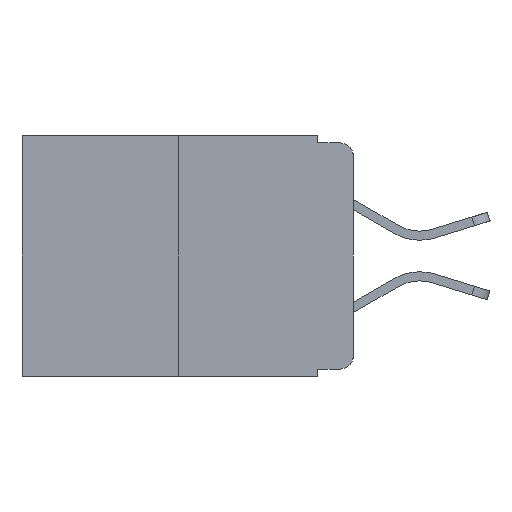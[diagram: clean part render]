
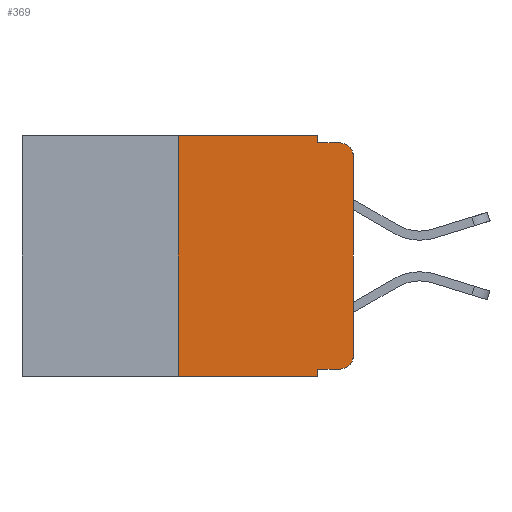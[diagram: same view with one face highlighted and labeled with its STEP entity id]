
A CAD part, left-side view. The second image highlights one B-rep face of the part: STEP entity #369.
In plain terms, the highlighted planar face has unit normal (-1, 0, 0).
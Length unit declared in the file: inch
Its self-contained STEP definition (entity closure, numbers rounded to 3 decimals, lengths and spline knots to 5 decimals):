
#134 = VERTEX_POINT ( 'NONE', #165 ) ;
#165 = CARTESIAN_POINT ( 'NONE',  ( 0., 0.051, 0. ) ) ;
#369 = ADVANCED_FACE ( 'NONE', ( #11028 ), #12728, .F. ) ;
#569 = LINE ( 'NONE', #6126, #7572 ) ;
#786 = VECTOR ( 'NONE', #8253, 39.37008 ) ;
#913 = VECTOR ( 'NONE', #2590, 39.37008 ) ;
#1004 = ORIENTED_EDGE ( 'NONE', *, *, #9226, .T. ) ;
#1346 = AXIS2_PLACEMENT_3D ( 'NONE', #11925, #11191, #14474 ) ;
#1442 = ORIENTED_EDGE ( 'NONE', *, *, #11062, .T. ) ;
#1674 = LINE ( 'NONE', #5457, #8709 ) ;
#1806 = EDGE_LOOP ( 'NONE', ( #15461, #11855, #4434, #7283, #9268, #16175, #1442, #15766, #1004, #14904 ) ) ;
#1819 = DIRECTION ( 'NONE',  ( 0., -1., 0. ) ) ;
#1820 = CARTESIAN_POINT ( 'NONE',  ( 0., 0.051, -0.333 ) ) ;
#1925 = DIRECTION ( 'NONE',  ( 1., 0., 0. ) ) ;
#2479 = VERTEX_POINT ( 'NONE', #3949 ) ;
#2590 = DIRECTION ( 'NONE',  ( 0., 0., 1. ) ) ;
#3297 = CARTESIAN_POINT ( 'NONE',  ( 0., 0.051, -0.01 ) ) ;
#3681 = EDGE_CURVE ( 'NONE', #13516, #15997, #10765, .T. ) ;
#3922 = EDGE_CURVE ( 'NONE', #4092, #17645, #17736, .T. ) ;
#3949 = CARTESIAN_POINT ( 'NONE',  ( 0., 0.25, -0.343 ) ) ;
#4070 = DIRECTION ( 'NONE',  ( -1., 0., 0. ) ) ;
#4092 = VERTEX_POINT ( 'NONE', #12322 ) ;
#4123 = CARTESIAN_POINT ( 'NONE',  ( 0., 0., 0. ) ) ;
#4226 = CARTESIAN_POINT ( 'NONE',  ( 0., 0.02, -0.313 ) ) ;
#4434 = ORIENTED_EDGE ( 'NONE', *, *, #15061, .F. ) ;
#4644 = LINE ( 'NONE', #4123, #913 ) ;
#4956 = LINE ( 'NONE', #17788, #786 ) ;
#5251 = CARTESIAN_POINT ( 'NONE',  ( 0., 0.473, 0. ) ) ;
#5457 = CARTESIAN_POINT ( 'NONE',  ( 0., 0.051, 0. ) ) ;
#5821 = EDGE_CURVE ( 'NONE', #134, #8652, #12830, .T. ) ;
#6102 = LINE ( 'NONE', #1820, #16618 ) ;
#6126 = CARTESIAN_POINT ( 'NONE',  ( 0., 0.473, -0.343 ) ) ;
#6387 = AXIS2_PLACEMENT_3D ( 'NONE', #4226, #4070, #17539 ) ;
#6771 = EDGE_CURVE ( 'NONE', #13102, #7600, #1674, .T. ) ;
#6887 = LINE ( 'NONE', #5251, #10620 ) ;
#7229 = EDGE_CURVE ( 'NONE', #15997, #4092, #4644, .T. ) ;
#7240 = CARTESIAN_POINT ( 'NONE',  ( 0., 0.02, -0.333 ) ) ;
#7283 = ORIENTED_EDGE ( 'NONE', *, *, #5821, .F. ) ;
#7415 = CARTESIAN_POINT ( 'NONE',  ( 0., 0.25, 0. ) ) ;
#7561 = CARTESIAN_POINT ( 'NONE',  ( 0., 0.051, -0.343 ) ) ;
#7572 = VECTOR ( 'NONE', #1819, 39.37008 ) ;
#7600 = VERTEX_POINT ( 'NONE', #7561 ) ;
#7799 = EDGE_CURVE ( 'NONE', #2479, #9155, #14393, .T. ) ;
#8253 = DIRECTION ( 'NONE',  ( 0., -1., 0. ) ) ;
#8652 = VERTEX_POINT ( 'NONE', #3297 ) ;
#8709 = VECTOR ( 'NONE', #11724, 39.37008 ) ;
#9155 = VERTEX_POINT ( 'NONE', #15509 ) ;
#9175 = VECTOR ( 'NONE', #15351, 39.37008 ) ;
#9226 = EDGE_CURVE ( 'NONE', #13102, #13516, #6102, .T. ) ;
#9268 = ORIENTED_EDGE ( 'NONE', *, *, #11332, .F. ) ;
#10620 = VECTOR ( 'NONE', #16263, 39.37008 ) ;
#10765 = CIRCLE ( 'NONE', #6387, 0.02 ) ;
#11028 = FACE_OUTER_BOUND ( 'NONE', #1806, .T. ) ;
#11062 = EDGE_CURVE ( 'NONE', #2479, #7600, #569, .T. ) ;
#11191 = DIRECTION ( 'NONE',  ( -1., 0., 0. ) ) ;
#11332 = EDGE_CURVE ( 'NONE', #9155, #134, #6887, .T. ) ;
#11724 = DIRECTION ( 'NONE',  ( 0., 0., -1. ) ) ;
#11855 = ORIENTED_EDGE ( 'NONE', *, *, #3922, .T. ) ;
#11925 = CARTESIAN_POINT ( 'NONE',  ( 0., 0.02, -0.03 ) ) ;
#12032 = DIRECTION ( 'NONE',  ( 0., 0., 1. ) ) ;
#12322 = CARTESIAN_POINT ( 'NONE',  ( 0., 0., -0.03 ) ) ;
#12728 = PLANE ( 'NONE',  #15118 ) ;
#12830 = LINE ( 'NONE', #13770, #9175 ) ;
#13102 = VERTEX_POINT ( 'NONE', #15980 ) ;
#13516 = VERTEX_POINT ( 'NONE', #7240 ) ;
#13770 = CARTESIAN_POINT ( 'NONE',  ( 0., 0.051, 0. ) ) ;
#13959 = VECTOR ( 'NONE', #12032, 39.37008 ) ;
#14393 = LINE ( 'NONE', #7415, #13959 ) ;
#14474 = DIRECTION ( 'NONE',  ( 0., 0., -1. ) ) ;
#14541 = CARTESIAN_POINT ( 'NONE',  ( 0., 0.02, -0.01 ) ) ;
#14904 = ORIENTED_EDGE ( 'NONE', *, *, #3681, .T. ) ;
#14931 = CARTESIAN_POINT ( 'NONE',  ( 0., 0.473, 0. ) ) ;
#15061 = EDGE_CURVE ( 'NONE', #8652, #17645, #4956, .T. ) ;
#15118 = AXIS2_PLACEMENT_3D ( 'NONE', #14931, #1925, #15162 ) ;
#15162 = DIRECTION ( 'NONE',  ( 0., 0., -1. ) ) ;
#15351 = DIRECTION ( 'NONE',  ( 0., 0., -1. ) ) ;
#15461 = ORIENTED_EDGE ( 'NONE', *, *, #7229, .T. ) ;
#15509 = CARTESIAN_POINT ( 'NONE',  ( 0., 0.25, 0. ) ) ;
#15766 = ORIENTED_EDGE ( 'NONE', *, *, #6771, .F. ) ;
#15851 = CARTESIAN_POINT ( 'NONE',  ( 0., 0., -0.313 ) ) ;
#15980 = CARTESIAN_POINT ( 'NONE',  ( 0., 0.051, -0.333 ) ) ;
#15997 = VERTEX_POINT ( 'NONE', #15851 ) ;
#16175 = ORIENTED_EDGE ( 'NONE', *, *, #7799, .F. ) ;
#16263 = DIRECTION ( 'NONE',  ( 0., -1., 0. ) ) ;
#16618 = VECTOR ( 'NONE', #17035, 39.37008 ) ;
#17035 = DIRECTION ( 'NONE',  ( 0., -1., 0. ) ) ;
#17539 = DIRECTION ( 'NONE',  ( 0., 0., -1. ) ) ;
#17645 = VERTEX_POINT ( 'NONE', #14541 ) ;
#17736 = CIRCLE ( 'NONE', #1346, 0.02 ) ;
#17788 = CARTESIAN_POINT ( 'NONE',  ( 0., 0.051, -0.01 ) ) ;
